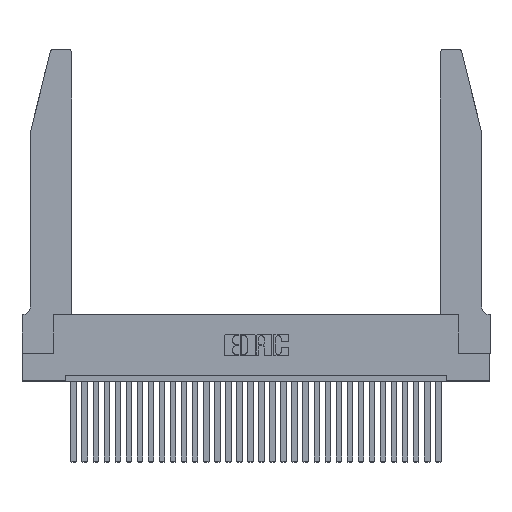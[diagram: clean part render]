
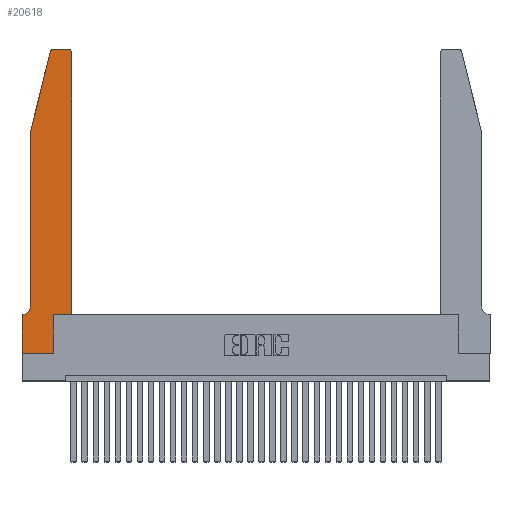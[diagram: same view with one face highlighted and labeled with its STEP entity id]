
A CAD part, top view. The second image highlights one B-rep face of the part: STEP entity #20618.
In plain terms, the highlighted planar face has unit normal (0, 0, 1).
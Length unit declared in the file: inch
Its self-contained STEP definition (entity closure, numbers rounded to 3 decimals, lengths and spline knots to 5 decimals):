
#1124 = VERTEX_POINT ( 'NONE', #30210 ) ;
#1354 = ORIENTED_EDGE ( 'NONE', *, *, #3627, .T. ) ;
#1526 = VECTOR ( 'NONE', #19660, 39.37008 ) ;
#1982 = EDGE_CURVE ( 'NONE', #25715, #8211, #13708, .T. ) ;
#2312 = VERTEX_POINT ( 'NONE', #9258 ) ;
#2522 = CARTESIAN_POINT ( 'NONE',  ( 0.0755, 0.42, 0.37 ) ) ;
#3076 = VERTEX_POINT ( 'NONE', #2522 ) ;
#3485 = DIRECTION ( 'NONE',  ( -1., 0., 0. ) ) ;
#3627 = EDGE_CURVE ( 'NONE', #1124, #16965, #16198, .T. ) ;
#3725 = EDGE_CURVE ( 'NONE', #14849, #7451, #23296, .T. ) ;
#4298 = ORIENTED_EDGE ( 'NONE', *, *, #23677, .T. ) ;
#4364 = DIRECTION ( 'NONE',  ( 0., 0., 1. ) ) ;
#4752 = LINE ( 'NONE', #29993, #26963 ) ;
#4832 = CARTESIAN_POINT ( 'NONE',  ( 0.2865, 0.35, 0.37 ) ) ;
#5173 = DIRECTION ( 'NONE',  ( 0., 0., 1. ) ) ;
#5228 = LINE ( 'NONE', #27067, #23281 ) ;
#5749 = DIRECTION ( 'NONE',  ( -1., 0., 0. ) ) ;
#6041 = EDGE_CURVE ( 'NONE', #15096, #25715, #5228, .T. ) ;
#6369 = EDGE_LOOP ( 'NONE', ( #20087, #12797, #1354, #27070, #4298, #27086, #14214, #27680, #20293, #20977, #24045, #24923 ) ) ;
#6562 = LINE ( 'NONE', #13722, #23861 ) ;
#6951 = CARTESIAN_POINT ( 'NONE',  ( 0., 0., 0.37 ) ) ;
#7451 = VERTEX_POINT ( 'NONE', #12669 ) ;
#8211 = VERTEX_POINT ( 'NONE', #25619 ) ;
#8453 = AXIS2_PLACEMENT_3D ( 'NONE', #31040, #4364, #14285 ) ;
#8989 = VECTOR ( 'NONE', #27668, 39.37008 ) ;
#9157 = CARTESIAN_POINT ( 'NONE',  ( 0., 0., 0.37 ) ) ;
#9258 = CARTESIAN_POINT ( 'NONE',  ( 0., 0.35, 0.37 ) ) ;
#9281 = CIRCLE ( 'NONE', #20340, 0.07 ) ;
#9572 = VERTEX_POINT ( 'NONE', #14227 ) ;
#9678 = VECTOR ( 'NONE', #3485, 39.37008 ) ;
#10646 = CARTESIAN_POINT ( 'NONE',  ( 0.2605, 2.75, 0.37 ) ) ;
#11437 = VECTOR ( 'NONE', #31082, 39.37008 ) ;
#11664 = LINE ( 'NONE', #15483, #8989 ) ;
#12317 = EDGE_CURVE ( 'NONE', #7451, #13117, #17947, .T. ) ;
#12475 = FACE_OUTER_BOUND ( 'NONE', #6369, .T. ) ;
#12669 = CARTESIAN_POINT ( 'NONE',  ( 0.4205, 2.75, 0.37 ) ) ;
#12770 = EDGE_CURVE ( 'NONE', #13117, #1124, #22761, .T. ) ;
#12797 = ORIENTED_EDGE ( 'NONE', *, *, #12770, .T. ) ;
#13117 = VERTEX_POINT ( 'NONE', #20995 ) ;
#13555 = CARTESIAN_POINT ( 'NONE',  ( 0.4205, 2.72, 0.37 ) ) ;
#13708 = LINE ( 'NONE', #4832, #19326 ) ;
#13722 = CARTESIAN_POINT ( 'NONE',  ( 0.0755, 2., 0.37 ) ) ;
#14122 = DIRECTION ( 'NONE',  ( 0., 1., 0. ) ) ;
#14214 = ORIENTED_EDGE ( 'NONE', *, *, #19240, .T. ) ;
#14227 = CARTESIAN_POINT ( 'NONE',  ( 0.0055, 0.35, 0.37 ) ) ;
#14285 = DIRECTION ( 'NONE',  ( 1., 0., 0. ) ) ;
#14849 = VERTEX_POINT ( 'NONE', #24562 ) ;
#15096 = VERTEX_POINT ( 'NONE', #9157 ) ;
#15346 = CARTESIAN_POINT ( 'NONE',  ( 0.2865, 0., 0.37 ) ) ;
#15483 = CARTESIAN_POINT ( 'NONE',  ( 0.4505, 0.35, 0.37 ) ) ;
#15918 = DIRECTION ( 'NONE',  ( -1., 0., 0. ) ) ;
#16198 = LINE ( 'NONE', #26720, #1526 ) ;
#16965 = VERTEX_POINT ( 'NONE', #23055 ) ;
#17037 = CARTESIAN_POINT ( 'NONE',  ( 0.4505, 0.35, 0.37 ) ) ;
#17152 = EDGE_CURVE ( 'NONE', #8211, #25675, #11664, .T. ) ;
#17460 = VECTOR ( 'NONE', #5749, 39.37008 ) ;
#17947 = LINE ( 'NONE', #10646, #9678 ) ;
#18956 = EDGE_CURVE ( 'NONE', #16965, #3076, #6562, .T. ) ;
#19240 = EDGE_CURVE ( 'NONE', #2312, #15096, #27614, .T. ) ;
#19326 = VECTOR ( 'NONE', #14122, 39.37008 ) ;
#19423 = EDGE_CURVE ( 'NONE', #9572, #2312, #26117, .T. ) ;
#19660 = DIRECTION ( 'NONE',  ( -0.239, -0.971, 0. ) ) ;
#19775 = CARTESIAN_POINT ( 'NONE',  ( 0., 0.35, 0.37 ) ) ;
#20087 = ORIENTED_EDGE ( 'NONE', *, *, #12317, .T. ) ;
#20293 = ORIENTED_EDGE ( 'NONE', *, *, #1982, .T. ) ;
#20340 = AXIS2_PLACEMENT_3D ( 'NONE', #25245, #25356, #15918 ) ;
#20618 = ADVANCED_FACE ( 'NONE', ( #12475 ), #24189, .T. ) ;
#20977 = ORIENTED_EDGE ( 'NONE', *, *, #17152, .T. ) ;
#20995 = CARTESIAN_POINT ( 'NONE',  ( 0.284, 2.75, 0.37 ) ) ;
#22180 = DIRECTION ( 'NONE',  ( 1., 0., 0. ) ) ;
#22756 = DIRECTION ( 'NONE',  ( 0., 1., 0. ) ) ;
#22761 = CIRCLE ( 'NONE', #8453, 0.03 ) ;
#23055 = CARTESIAN_POINT ( 'NONE',  ( 0.0755, 2., 0.37 ) ) ;
#23281 = VECTOR ( 'NONE', #24719, 39.37008 ) ;
#23296 = CIRCLE ( 'NONE', #29397, 0.03 ) ;
#23677 = EDGE_CURVE ( 'NONE', #3076, #9572, #9281, .T. ) ;
#23861 = VECTOR ( 'NONE', #30581, 39.37008 ) ;
#24045 = ORIENTED_EDGE ( 'NONE', *, *, #30024, .T. ) ;
#24189 = PLANE ( 'NONE',  #25729 ) ;
#24562 = CARTESIAN_POINT ( 'NONE',  ( 0.4505, 2.72, 0.37 ) ) ;
#24719 = DIRECTION ( 'NONE',  ( 1., 0., 0. ) ) ;
#24923 = ORIENTED_EDGE ( 'NONE', *, *, #3725, .T. ) ;
#25245 = CARTESIAN_POINT ( 'NONE',  ( 0.0055, 0.42, 0.37 ) ) ;
#25356 = DIRECTION ( 'NONE',  ( 0., 0., -1. ) ) ;
#25619 = CARTESIAN_POINT ( 'NONE',  ( 0.2865, 0.35, 0.37 ) ) ;
#25675 = VERTEX_POINT ( 'NONE', #17037 ) ;
#25715 = VERTEX_POINT ( 'NONE', #15346 ) ;
#25728 = DIRECTION ( 'NONE',  ( 1., 0., 0. ) ) ;
#25729 = AXIS2_PLACEMENT_3D ( 'NONE', #19775, #5173, #22180 ) ;
#26117 = LINE ( 'NONE', #29666, #17460 ) ;
#26720 = CARTESIAN_POINT ( 'NONE',  ( 0.0755, 2., 0.37 ) ) ;
#26963 = VECTOR ( 'NONE', #22756, 39.37008 ) ;
#27067 = CARTESIAN_POINT ( 'NONE',  ( 0., 0., 0.37 ) ) ;
#27070 = ORIENTED_EDGE ( 'NONE', *, *, #18956, .T. ) ;
#27086 = ORIENTED_EDGE ( 'NONE', *, *, #19423, .T. ) ;
#27614 = LINE ( 'NONE', #6951, #11437 ) ;
#27668 = DIRECTION ( 'NONE',  ( 1., 0., 0. ) ) ;
#27680 = ORIENTED_EDGE ( 'NONE', *, *, #6041, .T. ) ;
#29397 = AXIS2_PLACEMENT_3D ( 'NONE', #13555, #30202, #25728 ) ;
#29666 = CARTESIAN_POINT ( 'NONE',  ( 0.0755, 0.35, 0.37 ) ) ;
#29993 = CARTESIAN_POINT ( 'NONE',  ( 0.4505, 0.35, 0.37 ) ) ;
#30024 = EDGE_CURVE ( 'NONE', #25675, #14849, #4752, .T. ) ;
#30202 = DIRECTION ( 'NONE',  ( 0., 0., 1. ) ) ;
#30210 = CARTESIAN_POINT ( 'NONE',  ( 0.25487, 2.72718, 0.37 ) ) ;
#30581 = DIRECTION ( 'NONE',  ( 0., -1., 0. ) ) ;
#31040 = CARTESIAN_POINT ( 'NONE',  ( 0.284, 2.72, 0.37 ) ) ;
#31082 = DIRECTION ( 'NONE',  ( 0., -1., 0. ) ) ;
